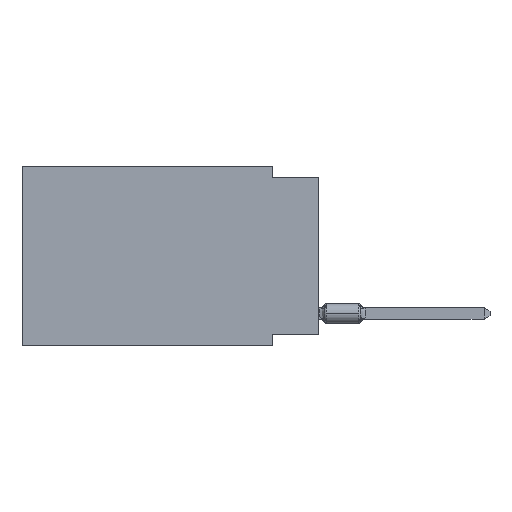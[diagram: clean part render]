
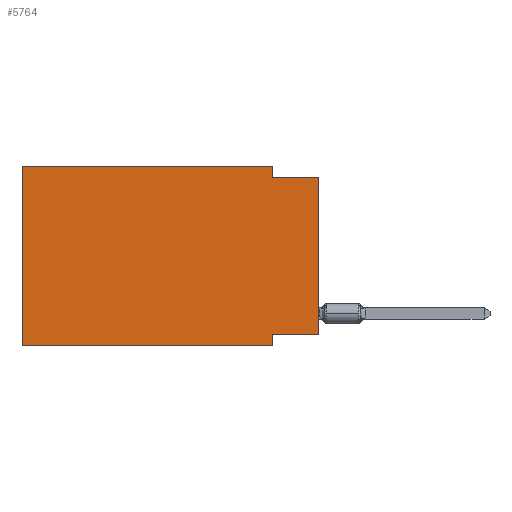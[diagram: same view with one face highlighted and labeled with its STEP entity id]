
A CAD part, left-side view. The second image highlights one B-rep face of the part: STEP entity #5764.
In plain terms, the highlighted planar face has unit normal (-1, 0, 0).
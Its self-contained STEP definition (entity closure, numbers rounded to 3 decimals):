
#289 = CARTESIAN_POINT ( 'NONE',  ( 0., 0., -0.635 ) ) ;
#472 = DIRECTION ( 'NONE',  ( 0., 0., -1. ) ) ;
#483 = VECTOR ( 'NONE', #628, 1000. ) ;
#628 = DIRECTION ( 'NONE',  ( 0., 1., 0. ) ) ;
#701 = VECTOR ( 'NONE', #9731, 1000. ) ;
#978 = VECTOR ( 'NONE', #13971, 1000. ) ;
#1123 = DIRECTION ( 'NONE',  ( 0., -1., 0. ) ) ;
#1660 = VERTEX_POINT ( 'NONE', #9873 ) ;
#1786 = LINE ( 'NONE', #6162, #978 ) ;
#1880 = EDGE_CURVE ( 'NONE', #7527, #9815, #11074, .T. ) ;
#1972 = LINE ( 'NONE', #13805, #8598 ) ;
#2053 = EDGE_CURVE ( 'NONE', #7504, #9815, #13439, .T. ) ;
#2503 = CARTESIAN_POINT ( 'NONE',  ( 0., 2.54, -9.271 ) ) ;
#3142 = CARTESIAN_POINT ( 'NONE',  ( 0., 2.54, -9.906 ) ) ;
#3294 = CARTESIAN_POINT ( 'NONE',  ( 0., 16.383, 0. ) ) ;
#3658 = VERTEX_POINT ( 'NONE', #10303 ) ;
#4073 = EDGE_LOOP ( 'NONE', ( #8758, #7105, #5923, #11924, #6022, #5106, #7596, #6484 ) ) ;
#4133 = CARTESIAN_POINT ( 'NONE',  ( 0., 0., -9.271 ) ) ;
#4226 = EDGE_CURVE ( 'NONE', #7527, #12315, #1972, .T. ) ;
#4638 = VECTOR ( 'NONE', #4822, 1000. ) ;
#4822 = DIRECTION ( 'NONE',  ( 0., 0., -1. ) ) ;
#5106 = ORIENTED_EDGE ( 'NONE', *, *, #1880, .T. ) ;
#5142 = CARTESIAN_POINT ( 'NONE',  ( 0., 16.383, -9.906 ) ) ;
#5427 = AXIS2_PLACEMENT_3D ( 'NONE', #11368, #13720, #472 ) ;
#5764 = ADVANCED_FACE ( 'NONE', ( #9346 ), #9205, .F. ) ;
#5923 = ORIENTED_EDGE ( 'NONE', *, *, #10055, .F. ) ;
#6022 = ORIENTED_EDGE ( 'NONE', *, *, #4226, .F. ) ;
#6162 = CARTESIAN_POINT ( 'NONE',  ( 0., 0., -0.635 ) ) ;
#6350 = DIRECTION ( 'NONE',  ( 0., 0., 1. ) ) ;
#6484 = ORIENTED_EDGE ( 'NONE', *, *, #14158, .F. ) ;
#7105 = ORIENTED_EDGE ( 'NONE', *, *, #13684, .F. ) ;
#7384 = VECTOR ( 'NONE', #1123, 1000. ) ;
#7504 = VERTEX_POINT ( 'NONE', #2503 ) ;
#7527 = VERTEX_POINT ( 'NONE', #5142 ) ;
#7546 = CARTESIAN_POINT ( 'NONE',  ( 0., 16.383, 0. ) ) ;
#7577 = DIRECTION ( 'NONE',  ( 0., 0., 1. ) ) ;
#7596 = ORIENTED_EDGE ( 'NONE', *, *, #2053, .F. ) ;
#8311 = LINE ( 'NONE', #12823, #10097 ) ;
#8589 = VERTEX_POINT ( 'NONE', #4133 ) ;
#8598 = VECTOR ( 'NONE', #6350, 1000. ) ;
#8758 = ORIENTED_EDGE ( 'NONE', *, *, #13170, .T. ) ;
#8972 = VECTOR ( 'NONE', #7577, 1000. ) ;
#9205 = PLANE ( 'NONE',  #5427 ) ;
#9346 = FACE_OUTER_BOUND ( 'NONE', #4073, .T. ) ;
#9731 = DIRECTION ( 'NONE',  ( 0., -1., 0. ) ) ;
#9815 = VERTEX_POINT ( 'NONE', #3142 ) ;
#9873 = CARTESIAN_POINT ( 'NONE',  ( 0., 2.54, 0. ) ) ;
#10030 = VERTEX_POINT ( 'NONE', #289 ) ;
#10055 = EDGE_CURVE ( 'NONE', #1660, #3658, #8311, .T. ) ;
#10063 = CARTESIAN_POINT ( 'NONE',  ( 0., 2.54, -9.906 ) ) ;
#10097 = VECTOR ( 'NONE', #12693, 1000. ) ;
#10303 = CARTESIAN_POINT ( 'NONE',  ( 0., 2.54, -0.635 ) ) ;
#10561 = CARTESIAN_POINT ( 'NONE',  ( 0., 0., -9.271 ) ) ;
#10856 = EDGE_CURVE ( 'NONE', #12315, #1660, #13970, .T. ) ;
#10929 = CARTESIAN_POINT ( 'NONE',  ( 0., 16.383, -9.906 ) ) ;
#10941 = CARTESIAN_POINT ( 'NONE',  ( 0., 0., 0. ) ) ;
#11074 = LINE ( 'NONE', #10929, #7384 ) ;
#11091 = LINE ( 'NONE', #10941, #8972 ) ;
#11368 = CARTESIAN_POINT ( 'NONE',  ( 0., 16.383, 0. ) ) ;
#11924 = ORIENTED_EDGE ( 'NONE', *, *, #10856, .F. ) ;
#12315 = VERTEX_POINT ( 'NONE', #7546 ) ;
#12693 = DIRECTION ( 'NONE',  ( 0., 0., -1. ) ) ;
#12823 = CARTESIAN_POINT ( 'NONE',  ( 0., 2.54, 0. ) ) ;
#13170 = EDGE_CURVE ( 'NONE', #8589, #10030, #11091, .T. ) ;
#13439 = LINE ( 'NONE', #10063, #4638 ) ;
#13684 = EDGE_CURVE ( 'NONE', #3658, #10030, #1786, .T. ) ;
#13720 = DIRECTION ( 'NONE',  ( 1., 0., 0. ) ) ;
#13805 = CARTESIAN_POINT ( 'NONE',  ( 0., 16.383, 0. ) ) ;
#13872 = LINE ( 'NONE', #10561, #483 ) ;
#13970 = LINE ( 'NONE', #3294, #701 ) ;
#13971 = DIRECTION ( 'NONE',  ( 0., -1., 0. ) ) ;
#14158 = EDGE_CURVE ( 'NONE', #8589, #7504, #13872, .T. ) ;
